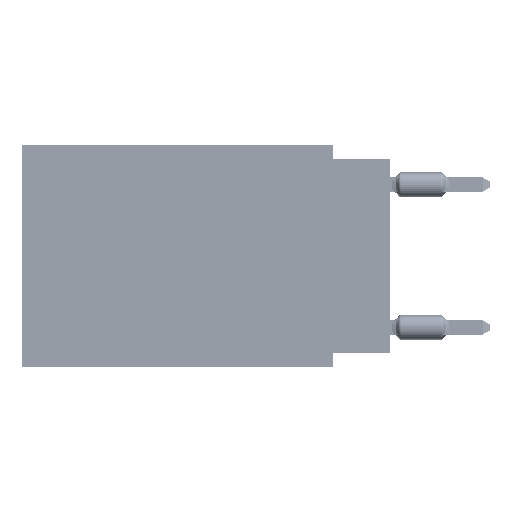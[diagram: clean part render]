
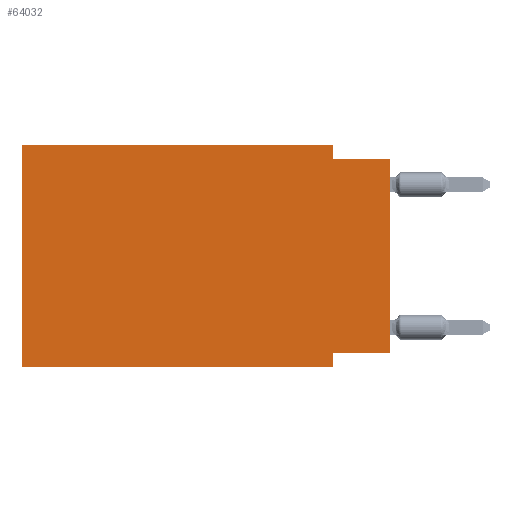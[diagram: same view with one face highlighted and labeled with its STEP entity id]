
A CAD part, left-side view. The second image highlights one B-rep face of the part: STEP entity #64032.
In plain terms, the highlighted planar face has unit normal (-1, 0, 0).
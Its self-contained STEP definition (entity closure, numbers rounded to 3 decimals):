
#346 = VERTEX_POINT ( 'NONE', #65078 ) ;
#849 = CARTESIAN_POINT ( 'NONE',  ( 0., 16.383, 0. ) ) ;
#2745 = CARTESIAN_POINT ( 'NONE',  ( 0., 0., -0.635 ) ) ;
#3971 = CARTESIAN_POINT ( 'NONE',  ( 0., 0., -9.271 ) ) ;
#5048 = EDGE_CURVE ( 'NONE', #44409, #29862, #9579, .T. ) ;
#6416 = VECTOR ( 'NONE', #59073, 1000. ) ;
#7193 = EDGE_CURVE ( 'NONE', #26249, #29862, #14778, .T. ) ;
#7562 = VECTOR ( 'NONE', #9430, 1000. ) ;
#7865 = DIRECTION ( 'NONE',  ( 0., -1., 0. ) ) ;
#8563 = ORIENTED_EDGE ( 'NONE', *, *, #52051, .T. ) ;
#9430 = DIRECTION ( 'NONE',  ( 0., 0., 1. ) ) ;
#9579 = LINE ( 'NONE', #21331, #6416 ) ;
#12285 = ORIENTED_EDGE ( 'NONE', *, *, #5048, .F. ) ;
#12762 = CARTESIAN_POINT ( 'NONE',  ( 0., 16.383, -9.906 ) ) ;
#14033 = ORIENTED_EDGE ( 'NONE', *, *, #67779, .F. ) ;
#14045 = CARTESIAN_POINT ( 'NONE',  ( 0., 16.383, 0. ) ) ;
#14778 = LINE ( 'NONE', #36487, #7562 ) ;
#15000 = DIRECTION ( 'NONE',  ( 0., 0., -1. ) ) ;
#18539 = CARTESIAN_POINT ( 'NONE',  ( 0., 16.383, 0. ) ) ;
#19865 = EDGE_CURVE ( 'NONE', #45796, #25284, #56653, .T. ) ;
#20055 = LINE ( 'NONE', #25036, #35531 ) ;
#21331 = CARTESIAN_POINT ( 'NONE',  ( 0., 0., -0.635 ) ) ;
#22770 = EDGE_CURVE ( 'NONE', #59400, #45796, #28601, .T. ) ;
#22778 = ORIENTED_EDGE ( 'NONE', *, *, #19865, .F. ) ;
#23702 = CARTESIAN_POINT ( 'NONE',  ( 0., 0., -9.271 ) ) ;
#24279 = DIRECTION ( 'NONE',  ( 0., 1., 0. ) ) ;
#25036 = CARTESIAN_POINT ( 'NONE',  ( 0., 2.54, 0. ) ) ;
#25284 = VERTEX_POINT ( 'NONE', #44527 ) ;
#26249 = VERTEX_POINT ( 'NONE', #23702 ) ;
#26882 = EDGE_LOOP ( 'NONE', ( #69417, #12285, #64741, #22778, #67737, #8563, #14033, #45353 ) ) ;
#28601 = LINE ( 'NONE', #849, #47791 ) ;
#29862 = VERTEX_POINT ( 'NONE', #2745 ) ;
#29969 = LINE ( 'NONE', #3971, #59341 ) ;
#30235 = EDGE_CURVE ( 'NONE', #26249, #346, #29969, .T. ) ;
#34918 = LINE ( 'NONE', #51641, #47295 ) ;
#35531 = VECTOR ( 'NONE', #52107, 1000. ) ;
#35762 = DIRECTION ( 'NONE',  ( 1., 0., 0. ) ) ;
#36487 = CARTESIAN_POINT ( 'NONE',  ( 0., 0., 0. ) ) ;
#41101 = FACE_OUTER_BOUND ( 'NONE', #26882, .T. ) ;
#43229 = VECTOR ( 'NONE', #15000, 1000. ) ;
#44409 = VERTEX_POINT ( 'NONE', #59900 ) ;
#44527 = CARTESIAN_POINT ( 'NONE',  ( 0., 2.54, 0. ) ) ;
#45190 = AXIS2_PLACEMENT_3D ( 'NONE', #14045, #35762, #59251 ) ;
#45353 = ORIENTED_EDGE ( 'NONE', *, *, #30235, .F. ) ;
#45796 = VERTEX_POINT ( 'NONE', #68864 ) ;
#47295 = VECTOR ( 'NONE', #67345, 1000. ) ;
#47791 = VECTOR ( 'NONE', #50319, 1000. ) ;
#48931 = VERTEX_POINT ( 'NONE', #50131 ) ;
#50131 = CARTESIAN_POINT ( 'NONE',  ( 0., 2.54, -9.906 ) ) ;
#50319 = DIRECTION ( 'NONE',  ( 0., 0., 1. ) ) ;
#51641 = CARTESIAN_POINT ( 'NONE',  ( 0., 16.383, -9.906 ) ) ;
#52051 = EDGE_CURVE ( 'NONE', #59400, #48931, #34918, .T. ) ;
#52107 = DIRECTION ( 'NONE',  ( 0., 0., -1. ) ) ;
#52191 = VECTOR ( 'NONE', #7865, 1000. ) ;
#54537 = EDGE_CURVE ( 'NONE', #25284, #44409, #20055, .T. ) ;
#56653 = LINE ( 'NONE', #18539, #52191 ) ;
#59073 = DIRECTION ( 'NONE',  ( 0., -1., 0. ) ) ;
#59251 = DIRECTION ( 'NONE',  ( 0., 0., -1. ) ) ;
#59341 = VECTOR ( 'NONE', #24279, 1000. ) ;
#59400 = VERTEX_POINT ( 'NONE', #12762 ) ;
#59900 = CARTESIAN_POINT ( 'NONE',  ( 0., 2.54, -0.635 ) ) ;
#62845 = PLANE ( 'NONE',  #45190 ) ;
#63097 = LINE ( 'NONE', #69853, #43229 ) ;
#64032 = ADVANCED_FACE ( 'NONE', ( #41101 ), #62845, .F. ) ;
#64741 = ORIENTED_EDGE ( 'NONE', *, *, #54537, .F. ) ;
#65078 = CARTESIAN_POINT ( 'NONE',  ( 0., 2.54, -9.271 ) ) ;
#67345 = DIRECTION ( 'NONE',  ( 0., -1., 0. ) ) ;
#67737 = ORIENTED_EDGE ( 'NONE', *, *, #22770, .F. ) ;
#67779 = EDGE_CURVE ( 'NONE', #346, #48931, #63097, .T. ) ;
#68864 = CARTESIAN_POINT ( 'NONE',  ( 0., 16.383, 0. ) ) ;
#69417 = ORIENTED_EDGE ( 'NONE', *, *, #7193, .T. ) ;
#69853 = CARTESIAN_POINT ( 'NONE',  ( 0., 2.54, -9.906 ) ) ;
